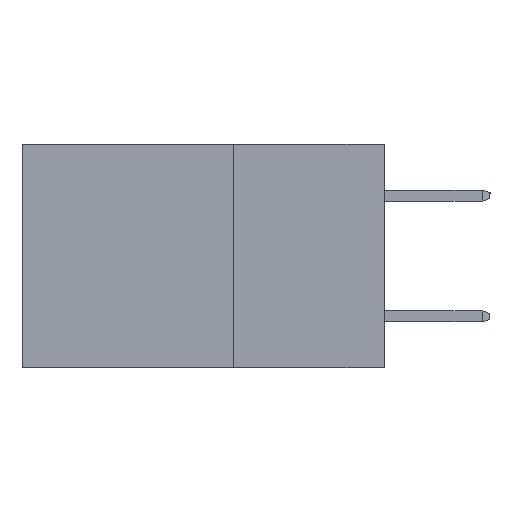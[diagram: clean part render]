
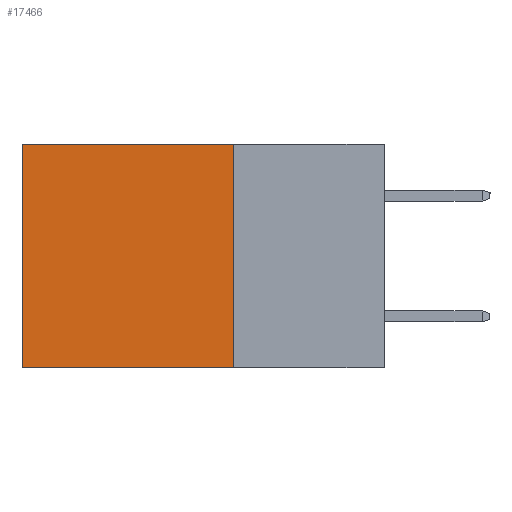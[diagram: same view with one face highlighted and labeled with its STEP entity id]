
A CAD part, left-side view. The second image highlights one B-rep face of the part: STEP entity #17466.
In plain terms, the highlighted planar face has unit normal (-1, 0, 0).
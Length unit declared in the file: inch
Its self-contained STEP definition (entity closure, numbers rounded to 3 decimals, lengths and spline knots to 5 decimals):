
#186 = EDGE_CURVE ( 'NONE', #14612, #10291, #732, .T. ) ;
#456 = ORIENTED_EDGE ( 'NONE', *, *, #17064, .F. ) ;
#732 = LINE ( 'NONE', #15084, #21408 ) ;
#744 = EDGE_CURVE ( 'NONE', #14556, #17218, #21723, .T. ) ;
#1150 = CARTESIAN_POINT ( 'NONE',  ( 0.2615, 0.6, 0. ) ) ;
#3643 = ORIENTED_EDGE ( 'NONE', *, *, #186, .F. ) ;
#5142 = VECTOR ( 'NONE', #15594, 39.37008 ) ;
#5531 = ORIENTED_EDGE ( 'NONE', *, *, #11095, .T. ) ;
#5956 = CARTESIAN_POINT ( 'NONE',  ( 0.2615, 0.6, -0.37 ) ) ;
#7928 = CARTESIAN_POINT ( 'NONE',  ( 0.2615, 0.25, 0. ) ) ;
#7947 = DIRECTION ( 'NONE',  ( 0., 0., -1. ) ) ;
#8474 = AXIS2_PLACEMENT_3D ( 'NONE', #17422, #19242, #8698 ) ;
#8698 = DIRECTION ( 'NONE',  ( 0., 0., -1. ) ) ;
#8885 = VECTOR ( 'NONE', #7947, 39.37008 ) ;
#9993 = ORIENTED_EDGE ( 'NONE', *, *, #744, .T. ) ;
#10291 = VERTEX_POINT ( 'NONE', #19436 ) ;
#10343 = CARTESIAN_POINT ( 'NONE',  ( 0.2615, 0.25, -0.37 ) ) ;
#10431 = FACE_OUTER_BOUND ( 'NONE', #18866, .T. ) ;
#11095 = EDGE_CURVE ( 'NONE', #14612, #14556, #14063, .T. ) ;
#11417 = DIRECTION ( 'NONE',  ( 0., 0., -1. ) ) ;
#14063 = LINE ( 'NONE', #15434, #17654 ) ;
#14556 = VERTEX_POINT ( 'NONE', #1150 ) ;
#14612 = VERTEX_POINT ( 'NONE', #7928 ) ;
#15084 = CARTESIAN_POINT ( 'NONE',  ( 0.2615, 0.25, -0.37 ) ) ;
#15434 = CARTESIAN_POINT ( 'NONE',  ( 0.2615, 0.25, 0. ) ) ;
#15594 = DIRECTION ( 'NONE',  ( 0., 1., 0. ) ) ;
#16554 = CARTESIAN_POINT ( 'NONE',  ( 0.2615, 0.6, -0.37 ) ) ;
#17064 = EDGE_CURVE ( 'NONE', #10291, #17218, #19366, .T. ) ;
#17218 = VERTEX_POINT ( 'NONE', #5956 ) ;
#17422 = CARTESIAN_POINT ( 'NONE',  ( 0.2615, 0.25, -0.37 ) ) ;
#17466 = ADVANCED_FACE ( 'NONE', ( #10431 ), #18909, .F. ) ;
#17654 = VECTOR ( 'NONE', #20814, 39.37008 ) ;
#18866 = EDGE_LOOP ( 'NONE', ( #9993, #456, #3643, #5531 ) ) ;
#18909 = PLANE ( 'NONE',  #8474 ) ;
#19242 = DIRECTION ( 'NONE',  ( 1., 0., 0. ) ) ;
#19366 = LINE ( 'NONE', #10343, #5142 ) ;
#19436 = CARTESIAN_POINT ( 'NONE',  ( 0.2615, 0.25, -0.37 ) ) ;
#20814 = DIRECTION ( 'NONE',  ( 0., 1., 0. ) ) ;
#21408 = VECTOR ( 'NONE', #11417, 39.37008 ) ;
#21723 = LINE ( 'NONE', #16554, #8885 ) ;
